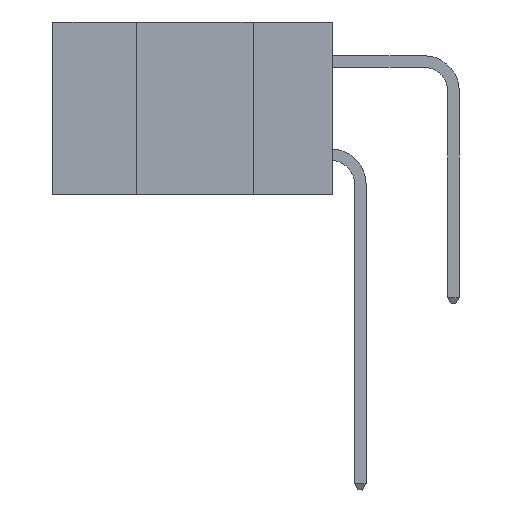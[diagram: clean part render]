
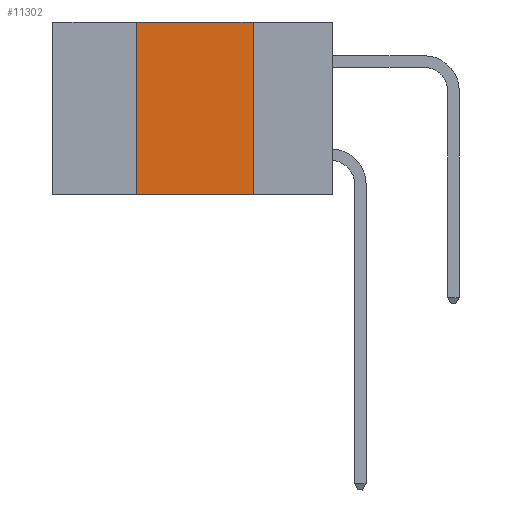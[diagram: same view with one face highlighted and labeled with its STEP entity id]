
A CAD part, left-side view. The second image highlights one B-rep face of the part: STEP entity #11302.
In plain terms, the highlighted planar face has unit normal (-1, 0, 0).
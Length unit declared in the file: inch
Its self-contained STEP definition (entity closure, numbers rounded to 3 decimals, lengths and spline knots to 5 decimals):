
#487 = ORIENTED_EDGE ( 'NONE', *, *, #14511, .F. ) ;
#962 = CARTESIAN_POINT ( 'NONE',  ( 0., 0.42, -0.37 ) ) ;
#994 = LINE ( 'NONE', #3241, #6145 ) ;
#1512 = VERTEX_POINT ( 'NONE', #962 ) ;
#1819 = VECTOR ( 'NONE', #9251, 39.37008 ) ;
#1926 = VECTOR ( 'NONE', #9854, 39.37008 ) ;
#3057 = VECTOR ( 'NONE', #10002, 39.37008 ) ;
#3241 = CARTESIAN_POINT ( 'NONE',  ( 0., 0.17, -0.37 ) ) ;
#3552 = CARTESIAN_POINT ( 'NONE',  ( 0., 0.6, 0. ) ) ;
#4256 = FACE_OUTER_BOUND ( 'NONE', #11433, .T. ) ;
#4407 = DIRECTION ( 'NONE',  ( 1., 0., 0. ) ) ;
#4554 = CARTESIAN_POINT ( 'NONE',  ( 0., 0.17, -0.37 ) ) ;
#4980 = CARTESIAN_POINT ( 'NONE',  ( 0., 0.42, 0. ) ) ;
#5095 = CARTESIAN_POINT ( 'NONE',  ( 0., 0.6, -0.37 ) ) ;
#5236 = CARTESIAN_POINT ( 'NONE',  ( 0., 0.42, -0.37 ) ) ;
#5481 = ORIENTED_EDGE ( 'NONE', *, *, #9190, .T. ) ;
#5701 = DIRECTION ( 'NONE',  ( 0., 0., -1. ) ) ;
#6145 = VECTOR ( 'NONE', #5701, 39.37008 ) ;
#6240 = LINE ( 'NONE', #5095, #1926 ) ;
#9110 = PLANE ( 'NONE',  #12838 ) ;
#9190 = EDGE_CURVE ( 'NONE', #1512, #10542, #6240, .T. ) ;
#9251 = DIRECTION ( 'NONE',  ( 0., -1., 0. ) ) ;
#9854 = DIRECTION ( 'NONE',  ( 0., -1., 0. ) ) ;
#10002 = DIRECTION ( 'NONE',  ( 0., 0., 1. ) ) ;
#10542 = VERTEX_POINT ( 'NONE', #4554 ) ;
#10592 = EDGE_CURVE ( 'NONE', #15156, #10542, #994, .T. ) ;
#10636 = LINE ( 'NONE', #3552, #1819 ) ;
#11030 = ORIENTED_EDGE ( 'NONE', *, *, #14125, .F. ) ;
#11302 = ADVANCED_FACE ( 'NONE', ( #4256 ), #9110, .F. ) ;
#11433 = EDGE_LOOP ( 'NONE', ( #13729, #11030, #487, #5481 ) ) ;
#11657 = DIRECTION ( 'NONE',  ( 0., 0., -1. ) ) ;
#11917 = CARTESIAN_POINT ( 'NONE',  ( 0., 0.17, 0. ) ) ;
#11941 = VERTEX_POINT ( 'NONE', #4980 ) ;
#12838 = AXIS2_PLACEMENT_3D ( 'NONE', #14910, #4407, #11657 ) ;
#13729 = ORIENTED_EDGE ( 'NONE', *, *, #10592, .F. ) ;
#14125 = EDGE_CURVE ( 'NONE', #11941, #15156, #10636, .T. ) ;
#14511 = EDGE_CURVE ( 'NONE', #1512, #11941, #14884, .T. ) ;
#14884 = LINE ( 'NONE', #5236, #3057 ) ;
#14910 = CARTESIAN_POINT ( 'NONE',  ( 0., 0.6, 0. ) ) ;
#15156 = VERTEX_POINT ( 'NONE', #11917 ) ;
